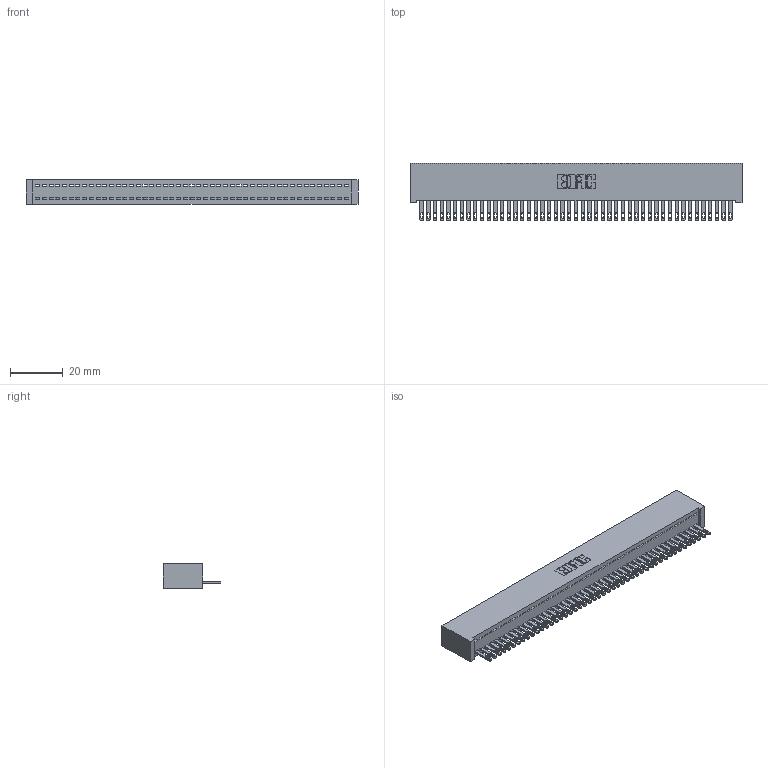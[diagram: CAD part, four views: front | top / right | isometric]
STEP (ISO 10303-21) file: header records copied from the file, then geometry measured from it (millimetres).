
FILE_DESCRIPTION (( 'STEP AP203' ), '1' );
FILE_NAME ('892-047-500-101.STEP', '2020-09-21T17:21:34', ( '' ), ( '' ), 'SwSTEP 2.0', 'SolidWorks 2020', '' );
FILE_SCHEMA (( 'CONFIG_CONTROL_DESIGN' ));
Length unit declared in the file: inch
Products named in the file (3): 345-292-001_345-293-100; 892-047-500-101; 842 Part_Lugless
Assembly tree (48 placements, depth 2):
  892-047-500-101
    842 Part_Lugless
    345-292-001_345-293-100  x47
Bounding box: 125.63 x 21.85 x 9.4 mm (x, y, z)
Volume: 11471.6 mm3; surface area: 17354.7 mm2
Topology: 48 solids, 48 shells, 2640 faces, 8171 edges, 5446 vertices
Faces by surface type: plane 1754, cylinder 886
Entity records: 27607 total; most frequent: CARTESIAN_POINT 4767, ORIENTED_EDGE 4750, DIRECTION 4005, EDGE_CURVE 2375, LINE 2251, VECTOR 2251, VERTEX_POINT 1582, AXIS2_PLACEMENT_3D 877
